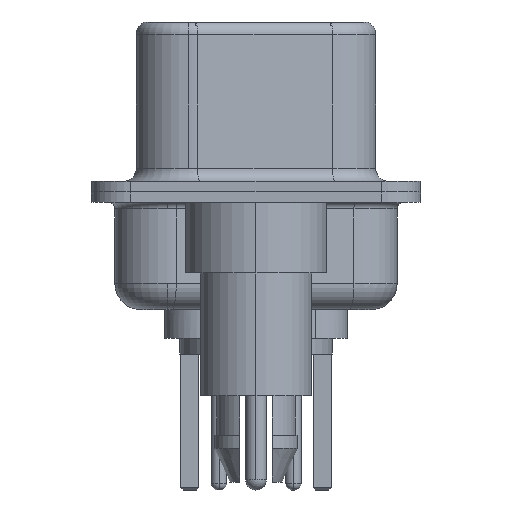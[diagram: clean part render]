
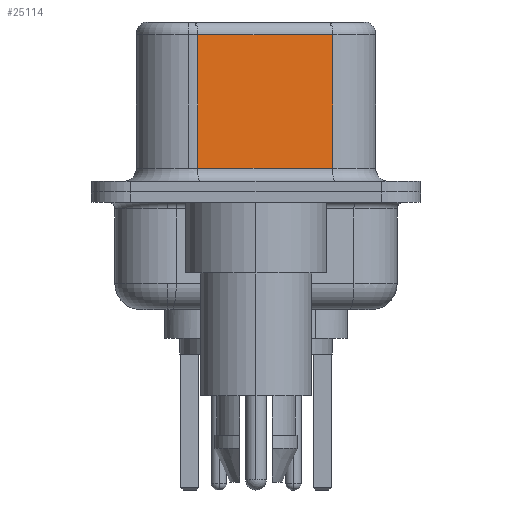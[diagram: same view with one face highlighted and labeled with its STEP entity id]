
A CAD part, left-side view. The second image highlights one B-rep face of the part: STEP entity #25114.
In plain terms, the highlighted planar face has unit normal (-0.985, -0.174, 0).
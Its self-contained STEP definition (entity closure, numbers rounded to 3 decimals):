
#271 = CARTESIAN_POINT ( 'NONE',  ( 4.58, -2.927, 6.52 ) ) ;
#550 = LINE ( 'NONE', #15873, #21365 ) ;
#900 = LINE ( 'NONE', #4993, #15716 ) ;
#1925 = ORIENTED_EDGE ( 'NONE', *, *, #17321, .T. ) ;
#2074 = VERTEX_POINT ( 'NONE', #7433 ) ;
#4397 = DIRECTION ( 'NONE',  ( -0.174, 0.985, 0. ) ) ;
#4993 = CARTESIAN_POINT ( 'NONE',  ( 4.58, -2.927, 0.9 ) ) ;
#5198 = VERTEX_POINT ( 'NONE', #6407 ) ;
#5332 = ORIENTED_EDGE ( 'NONE', *, *, #16872, .F. ) ;
#6407 = CARTESIAN_POINT ( 'NONE',  ( 3.67, 2.233, 6.02 ) ) ;
#6508 = CARTESIAN_POINT ( 'NONE',  ( 4.58, -2.927, 0.9 ) ) ;
#7433 = CARTESIAN_POINT ( 'NONE',  ( 3.67, 2.233, 0.9 ) ) ;
#9075 = DIRECTION ( 'NONE',  ( -0.174, 0.985, 0. ) ) ;
#9107 = ORIENTED_EDGE ( 'NONE', *, *, #16066, .T. ) ;
#9377 = CARTESIAN_POINT ( 'NONE',  ( 4.58, -2.927, 6.52 ) ) ;
#9838 = VERTEX_POINT ( 'NONE', #15129 ) ;
#13393 = FACE_OUTER_BOUND ( 'NONE', #25516, .T. ) ;
#14420 = PLANE ( 'NONE',  #20517 ) ;
#15129 = CARTESIAN_POINT ( 'NONE',  ( 4.58, -2.927, 6.02 ) ) ;
#15716 = VECTOR ( 'NONE', #21110, 1000. ) ;
#15873 = CARTESIAN_POINT ( 'NONE',  ( 3.67, 2.233, 6.52 ) ) ;
#16066 = EDGE_CURVE ( 'NONE', #9838, #5198, #25575, .T. ) ;
#16470 = DIRECTION ( 'NONE',  ( 0.985, 0.174, 0. ) ) ;
#16872 = EDGE_CURVE ( 'NONE', #9838, #19293, #25218, .T. ) ;
#17321 = EDGE_CURVE ( 'NONE', #2074, #19293, #900, .T. ) ;
#18027 = EDGE_CURVE ( 'NONE', #5198, #2074, #550, .T. ) ;
#19293 = VERTEX_POINT ( 'NONE', #6508 ) ;
#19550 = VECTOR ( 'NONE', #9075, 1000. ) ;
#19842 = VECTOR ( 'NONE', #23590, 1000. ) ;
#20517 = AXIS2_PLACEMENT_3D ( 'NONE', #271, #16470, #4397 ) ;
#21110 = DIRECTION ( 'NONE',  ( 0.174, -0.985, 0. ) ) ;
#21365 = VECTOR ( 'NONE', #21957, 1000. ) ;
#21957 = DIRECTION ( 'NONE',  ( 0., 0., -1. ) ) ;
#22439 = ORIENTED_EDGE ( 'NONE', *, *, #18027, .T. ) ;
#23202 = CARTESIAN_POINT ( 'NONE',  ( 4.58, -2.927, 6.02 ) ) ;
#23590 = DIRECTION ( 'NONE',  ( 0., 0., -1. ) ) ;
#25114 = ADVANCED_FACE ( 'NONE', ( #13393 ), #14420, .F. ) ;
#25218 = LINE ( 'NONE', #9377, #19842 ) ;
#25516 = EDGE_LOOP ( 'NONE', ( #5332, #9107, #22439, #1925 ) ) ;
#25575 = LINE ( 'NONE', #23202, #19550 ) ;
